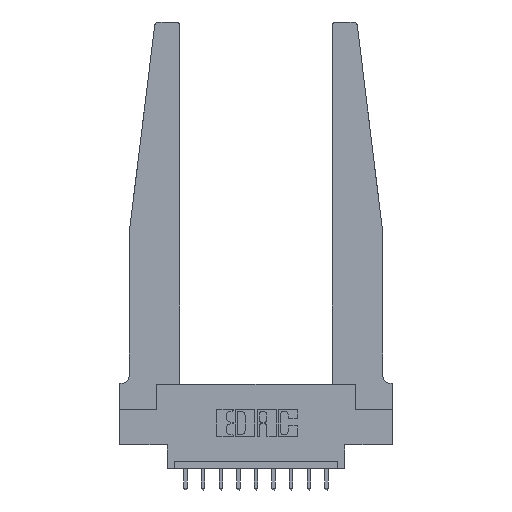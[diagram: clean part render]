
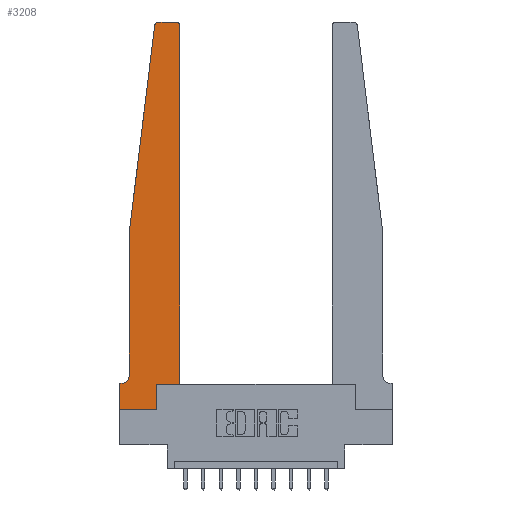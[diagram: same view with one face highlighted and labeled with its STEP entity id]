
A CAD part, top view. The second image highlights one B-rep face of the part: STEP entity #3208.
In plain terms, the highlighted planar face has unit normal (0, 0, 1).
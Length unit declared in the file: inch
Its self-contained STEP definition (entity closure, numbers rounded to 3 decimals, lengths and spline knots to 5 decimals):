
#46 = VECTOR ( 'NONE', #8838, 39.37008 ) ;
#403 = CARTESIAN_POINT ( 'NONE',  ( 0.27653, 2.72, 0.37 ) ) ;
#431 = DIRECTION ( 'NONE',  ( -1., 0., 0. ) ) ;
#528 = VERTEX_POINT ( 'NONE', #13456 ) ;
#551 = EDGE_CURVE ( 'NONE', #13982, #3446, #8919, .T. ) ;
#574 = ORIENTED_EDGE ( 'NONE', *, *, #12040, .T. ) ;
#587 = ORIENTED_EDGE ( 'NONE', *, *, #2064, .T. ) ;
#649 = CARTESIAN_POINT ( 'NONE',  ( 0.395, 2.75, 0.37 ) ) ;
#718 = DIRECTION ( 'NONE',  ( 1., 0., 0. ) ) ;
#761 = EDGE_CURVE ( 'NONE', #6084, #13995, #2781, .T. ) ;
#849 = CARTESIAN_POINT ( 'NONE',  ( 0., 0., 0.37 ) ) ;
#923 = ORIENTED_EDGE ( 'NONE', *, *, #10517, .T. ) ;
#1494 = ORIENTED_EDGE ( 'NONE', *, *, #4046, .T. ) ;
#1542 = LINE ( 'NONE', #5556, #4527 ) ;
#2064 = EDGE_CURVE ( 'NONE', #13995, #6297, #1542, .T. ) ;
#2111 = LINE ( 'NONE', #12743, #7562 ) ;
#2285 = VECTOR ( 'NONE', #4638, 39.37008 ) ;
#2340 = DIRECTION ( 'NONE',  ( 0., 1., 0. ) ) ;
#2516 = PLANE ( 'NONE',  #14389 ) ;
#2738 = VERTEX_POINT ( 'NONE', #4130 ) ;
#2781 = LINE ( 'NONE', #7461, #10930 ) ;
#3208 = ADVANCED_FACE ( 'NONE', ( #13154 ), #2516, .T. ) ;
#3446 = VERTEX_POINT ( 'NONE', #9703 ) ;
#3756 = DIRECTION ( 'NONE',  ( -1., 0., 0. ) ) ;
#3911 = DIRECTION ( 'NONE',  ( 0., 0., -1. ) ) ;
#4040 = CARTESIAN_POINT ( 'NONE',  ( 0.24675, 2.72367, 0.37 ) ) ;
#4046 = EDGE_CURVE ( 'NONE', #528, #6084, #5678, .T. ) ;
#4129 = DIRECTION ( 'NONE',  ( 0., 0., 1. ) ) ;
#4130 = CARTESIAN_POINT ( 'NONE',  ( 0.425, 2.72, 0.37 ) ) ;
#4232 = AXIS2_PLACEMENT_3D ( 'NONE', #14499, #3911, #9961 ) ;
#4527 = VECTOR ( 'NONE', #10466, 39.37008 ) ;
#4596 = VERTEX_POINT ( 'NONE', #13063 ) ;
#4638 = DIRECTION ( 'NONE',  ( 0., -1., 0. ) ) ;
#4666 = CARTESIAN_POINT ( 'NONE',  ( 0.395, 2.72, 0.37 ) ) ;
#4898 = VECTOR ( 'NONE', #2340, 39.37008 ) ;
#5003 = CARTESIAN_POINT ( 'NONE',  ( 0., 0.1875, 0.37 ) ) ;
#5152 = DIRECTION ( 'NONE',  ( 1., 0., 0. ) ) ;
#5376 = ORIENTED_EDGE ( 'NONE', *, *, #14898, .T. ) ;
#5482 = ORIENTED_EDGE ( 'NONE', *, *, #761, .T. ) ;
#5524 = CARTESIAN_POINT ( 'NONE',  ( 0.065, 1.25, 0.37 ) ) ;
#5556 = CARTESIAN_POINT ( 'NONE',  ( 0.065, 1.25, 0.37 ) ) ;
#5581 = ORIENTED_EDGE ( 'NONE', *, *, #7968, .T. ) ;
#5584 = ORIENTED_EDGE ( 'NONE', *, *, #551, .T. ) ;
#5678 = CIRCLE ( 'NONE', #8928, 0.03 ) ;
#5931 = CIRCLE ( 'NONE', #4232, 0.05 ) ;
#6061 = ORIENTED_EDGE ( 'NONE', *, *, #6943, .T. ) ;
#6084 = VERTEX_POINT ( 'NONE', #4040 ) ;
#6239 = CARTESIAN_POINT ( 'NONE',  ( 0.425, 0.18, 0.37 ) ) ;
#6297 = VERTEX_POINT ( 'NONE', #9190 ) ;
#6943 = EDGE_CURVE ( 'NONE', #3446, #15016, #2111, .T. ) ;
#7190 = CARTESIAN_POINT ( 'NONE',  ( 0., 0.1875, 0.37 ) ) ;
#7214 = CARTESIAN_POINT ( 'NONE',  ( 0.425, 0.18, 0.37 ) ) ;
#7252 = CARTESIAN_POINT ( 'NONE',  ( 0.425, 0.18, 0.37 ) ) ;
#7430 = VERTEX_POINT ( 'NONE', #5003 ) ;
#7461 = CARTESIAN_POINT ( 'NONE',  ( 0.065, 1.25, 0.37 ) ) ;
#7562 = VECTOR ( 'NONE', #13879, 39.37008 ) ;
#7968 = EDGE_CURVE ( 'NONE', #2738, #8728, #10562, .T. ) ;
#8181 = VECTOR ( 'NONE', #3756, 39.37008 ) ;
#8426 = LINE ( 'NONE', #7214, #14168 ) ;
#8630 = CARTESIAN_POINT ( 'NONE',  ( 0.065, 0.1875, 0.37 ) ) ;
#8728 = VERTEX_POINT ( 'NONE', #649 ) ;
#8754 = ORIENTED_EDGE ( 'NONE', *, *, #8764, .T. ) ;
#8764 = EDGE_CURVE ( 'NONE', #4596, #7430, #8863, .T. ) ;
#8838 = DIRECTION ( 'NONE',  ( 1., 0., 0. ) ) ;
#8863 = LINE ( 'NONE', #8630, #14931 ) ;
#8919 = LINE ( 'NONE', #849, #46 ) ;
#8928 = AXIS2_PLACEMENT_3D ( 'NONE', #403, #13458, #9553 ) ;
#9190 = CARTESIAN_POINT ( 'NONE',  ( 0.065, 0.2375, 0.37 ) ) ;
#9302 = LINE ( 'NONE', #10539, #2285 ) ;
#9459 = VERTEX_POINT ( 'NONE', #6239 ) ;
#9553 = DIRECTION ( 'NONE',  ( 1., 0., 0. ) ) ;
#9703 = CARTESIAN_POINT ( 'NONE',  ( 0.2605, 0., 0.37 ) ) ;
#9961 = DIRECTION ( 'NONE',  ( -1., 0., 0. ) ) ;
#10386 = CARTESIAN_POINT ( 'NONE',  ( 0.2605, 0.18, 0.37 ) ) ;
#10404 = EDGE_CURVE ( 'NONE', #6297, #4596, #5931, .T. ) ;
#10463 = EDGE_LOOP ( 'NONE', ( #11592, #1494, #5482, #587, #15260, #8754, #574, #5584, #6061, #923, #5376, #5581 ) ) ;
#10466 = DIRECTION ( 'NONE',  ( 0., -1., 0. ) ) ;
#10517 = EDGE_CURVE ( 'NONE', #15016, #9459, #8426, .T. ) ;
#10539 = CARTESIAN_POINT ( 'NONE',  ( 0., 0., 0.37 ) ) ;
#10562 = CIRCLE ( 'NONE', #13578, 0.03 ) ;
#10799 = LINE ( 'NONE', #7252, #4898 ) ;
#10930 = VECTOR ( 'NONE', #14601, 39.37008 ) ;
#10999 = EDGE_CURVE ( 'NONE', #8728, #528, #12133, .T. ) ;
#11592 = ORIENTED_EDGE ( 'NONE', *, *, #10999, .T. ) ;
#11812 = DIRECTION ( 'NONE',  ( 1., 0., 0. ) ) ;
#12040 = EDGE_CURVE ( 'NONE', #7430, #13982, #9302, .T. ) ;
#12133 = LINE ( 'NONE', #14426, #8181 ) ;
#12743 = CARTESIAN_POINT ( 'NONE',  ( 0.2605, 0.18, 0.37 ) ) ;
#13063 = CARTESIAN_POINT ( 'NONE',  ( 0.015, 0.1875, 0.37 ) ) ;
#13136 = DIRECTION ( 'NONE',  ( 0., 0., 1. ) ) ;
#13154 = FACE_OUTER_BOUND ( 'NONE', #10463, .T. ) ;
#13456 = CARTESIAN_POINT ( 'NONE',  ( 0.27653, 2.75, 0.37 ) ) ;
#13458 = DIRECTION ( 'NONE',  ( 0., 0., 1. ) ) ;
#13578 = AXIS2_PLACEMENT_3D ( 'NONE', #4666, #13136, #11812 ) ;
#13879 = DIRECTION ( 'NONE',  ( 0., 1., 0. ) ) ;
#13959 = CARTESIAN_POINT ( 'NONE',  ( 0., 0., 0.37 ) ) ;
#13982 = VERTEX_POINT ( 'NONE', #13959 ) ;
#13995 = VERTEX_POINT ( 'NONE', #5524 ) ;
#14168 = VECTOR ( 'NONE', #5152, 39.37008 ) ;
#14389 = AXIS2_PLACEMENT_3D ( 'NONE', #7190, #4129, #718 ) ;
#14426 = CARTESIAN_POINT ( 'NONE',  ( 0.25, 2.75, 0.37 ) ) ;
#14499 = CARTESIAN_POINT ( 'NONE',  ( 0.015, 0.2375, 0.37 ) ) ;
#14601 = DIRECTION ( 'NONE',  ( -0.122, -0.992, 0. ) ) ;
#14898 = EDGE_CURVE ( 'NONE', #9459, #2738, #10799, .T. ) ;
#14931 = VECTOR ( 'NONE', #431, 39.37008 ) ;
#15016 = VERTEX_POINT ( 'NONE', #10386 ) ;
#15260 = ORIENTED_EDGE ( 'NONE', *, *, #10404, .T. ) ;
